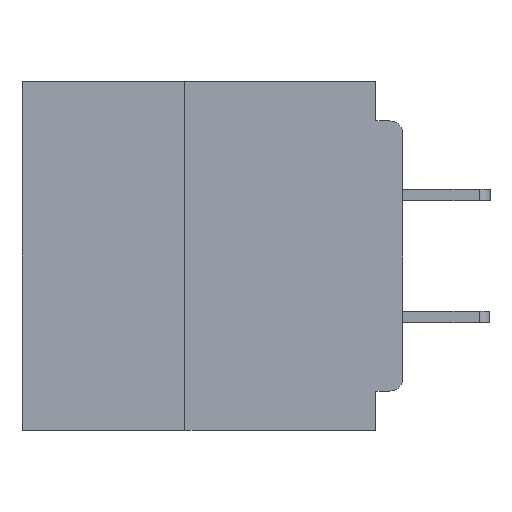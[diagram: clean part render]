
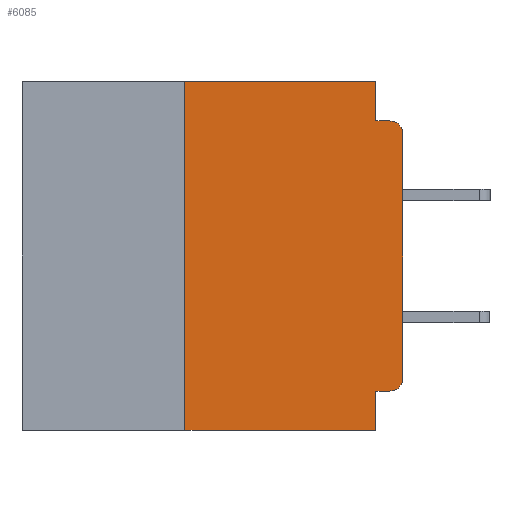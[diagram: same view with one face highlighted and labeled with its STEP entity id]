
A CAD part, left-side view. The second image highlights one B-rep face of the part: STEP entity #6085.
In plain terms, the highlighted planar face has unit normal (-1, 0, 0).
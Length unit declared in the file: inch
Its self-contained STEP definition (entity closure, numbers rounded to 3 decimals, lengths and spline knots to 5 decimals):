
#209 = LINE ( 'NONE', #24996, #17681 ) ;
#432 = CARTESIAN_POINT ( 'NONE',  ( 0., 0.015, -0.045 ) ) ;
#814 = VECTOR ( 'NONE', #6378, 39.37008 ) ;
#1508 = EDGE_CURVE ( 'NONE', #24689, #15561, #11261, .T. ) ;
#1944 = EDGE_CURVE ( 'NONE', #20223, #42986, #40519, .T. ) ;
#2173 = VECTOR ( 'NONE', #44074, 39.37008 ) ;
#2758 = CARTESIAN_POINT ( 'NONE',  ( 0., 0.437, -0.4 ) ) ;
#2955 = CARTESIAN_POINT ( 'NONE',  ( 0., 0.015, -0.355 ) ) ;
#4471 = VECTOR ( 'NONE', #29755, 39.37008 ) ;
#5845 = CARTESIAN_POINT ( 'NONE',  ( 0., 0.25, 0. ) ) ;
#6073 = CARTESIAN_POINT ( 'NONE',  ( 0., 0.015, -0.06 ) ) ;
#6085 = ADVANCED_FACE ( 'NONE', ( #31059 ), #6500, .F. ) ;
#6378 = DIRECTION ( 'NONE',  ( 0., 1., 0. ) ) ;
#6500 = PLANE ( 'NONE',  #25176 ) ;
#6593 = CARTESIAN_POINT ( 'NONE',  ( 0., 0., -0.355 ) ) ;
#7092 = LINE ( 'NONE', #2758, #25419 ) ;
#7213 = ORIENTED_EDGE ( 'NONE', *, *, #21589, .T. ) ;
#7662 = CARTESIAN_POINT ( 'NONE',  ( 0., 0., -0.06 ) ) ;
#9269 = CARTESIAN_POINT ( 'NONE',  ( 0., 0.437, 0. ) ) ;
#9565 = DIRECTION ( 'NONE',  ( 0., 0., -1. ) ) ;
#9744 = CIRCLE ( 'NONE', #31166, 0.015 ) ;
#9876 = VERTEX_POINT ( 'NONE', #36592 ) ;
#9993 = DIRECTION ( 'NONE',  ( 1., 0., 0. ) ) ;
#10496 = EDGE_CURVE ( 'NONE', #26875, #34018, #22851, .T. ) ;
#11261 = LINE ( 'NONE', #6593, #814 ) ;
#11410 = EDGE_CURVE ( 'NONE', #15561, #9876, #30737, .T. ) ;
#11480 = LINE ( 'NONE', #43930, #2173 ) ;
#12088 = VECTOR ( 'NONE', #33208, 39.37008 ) ;
#15561 = VERTEX_POINT ( 'NONE', #44194 ) ;
#16716 = DIRECTION ( 'NONE',  ( 0., 0., -1. ) ) ;
#17394 = VERTEX_POINT ( 'NONE', #41578 ) ;
#17456 = EDGE_CURVE ( 'NONE', #17394, #35552, #209, .T. ) ;
#17681 = VECTOR ( 'NONE', #28429, 39.37008 ) ;
#19764 = EDGE_CURVE ( 'NONE', #35552, #20223, #30267, .T. ) ;
#20223 = VERTEX_POINT ( 'NONE', #32751 ) ;
#20227 = CARTESIAN_POINT ( 'NONE',  ( 0., 0.437, 0. ) ) ;
#20500 = CARTESIAN_POINT ( 'NONE',  ( 0., 0.015, -0.34 ) ) ;
#20991 = EDGE_CURVE ( 'NONE', #17394, #9876, #7092, .T. ) ;
#21589 = EDGE_CURVE ( 'NONE', #34018, #39240, #9744, .T. ) ;
#21604 = CARTESIAN_POINT ( 'NONE',  ( 0., 0.031, 0. ) ) ;
#22851 = LINE ( 'NONE', #43211, #4471 ) ;
#23958 = DIRECTION ( 'NONE',  ( 0., 0., -1. ) ) ;
#24314 = AXIS2_PLACEMENT_3D ( 'NONE', #20500, #44247, #23958 ) ;
#24689 = VERTEX_POINT ( 'NONE', #2955 ) ;
#24996 = CARTESIAN_POINT ( 'NONE',  ( 0., 0.25, -0.4 ) ) ;
#25176 = AXIS2_PLACEMENT_3D ( 'NONE', #20227, #9993, #33913 ) ;
#25419 = VECTOR ( 'NONE', #36936, 39.37008 ) ;
#26376 = CIRCLE ( 'NONE', #24314, 0.015 ) ;
#26875 = VERTEX_POINT ( 'NONE', #36315 ) ;
#27724 = CARTESIAN_POINT ( 'NONE',  ( 0., 0.031, -0.045 ) ) ;
#27869 = ORIENTED_EDGE ( 'NONE', *, *, #20991, .T. ) ;
#27899 = ORIENTED_EDGE ( 'NONE', *, *, #1944, .F. ) ;
#28429 = DIRECTION ( 'NONE',  ( 0., 0., 1. ) ) ;
#29681 = VECTOR ( 'NONE', #16716, 39.37008 ) ;
#29755 = DIRECTION ( 'NONE',  ( 0., 0., 1. ) ) ;
#30113 = DIRECTION ( 'NONE',  ( -1., 0., 0. ) ) ;
#30267 = LINE ( 'NONE', #9269, #12088 ) ;
#30483 = VECTOR ( 'NONE', #41935, 39.37008 ) ;
#30646 = EDGE_CURVE ( 'NONE', #42986, #39240, #11480, .T. ) ;
#30737 = LINE ( 'NONE', #43900, #29681 ) ;
#31059 = FACE_OUTER_BOUND ( 'NONE', #42740, .T. ) ;
#31166 = AXIS2_PLACEMENT_3D ( 'NONE', #6073, #30113, #9565 ) ;
#32751 = CARTESIAN_POINT ( 'NONE',  ( 0., 0.031, 0. ) ) ;
#33208 = DIRECTION ( 'NONE',  ( 0., -1., 0. ) ) ;
#33913 = DIRECTION ( 'NONE',  ( 0., 0., -1. ) ) ;
#34018 = VERTEX_POINT ( 'NONE', #7662 ) ;
#35078 = ORIENTED_EDGE ( 'NONE', *, *, #17456, .F. ) ;
#35552 = VERTEX_POINT ( 'NONE', #5845 ) ;
#36315 = CARTESIAN_POINT ( 'NONE',  ( 0., 0., -0.34 ) ) ;
#36592 = CARTESIAN_POINT ( 'NONE',  ( 0., 0.031, -0.4 ) ) ;
#36936 = DIRECTION ( 'NONE',  ( 0., -1., 0. ) ) ;
#37521 = ORIENTED_EDGE ( 'NONE', *, *, #10496, .T. ) ;
#37665 = ORIENTED_EDGE ( 'NONE', *, *, #40474, .T. ) ;
#39240 = VERTEX_POINT ( 'NONE', #432 ) ;
#39669 = ORIENTED_EDGE ( 'NONE', *, *, #19764, .F. ) ;
#40474 = EDGE_CURVE ( 'NONE', #24689, #26875, #26376, .T. ) ;
#40519 = LINE ( 'NONE', #21604, #30483 ) ;
#40814 = ORIENTED_EDGE ( 'NONE', *, *, #11410, .F. ) ;
#41536 = ORIENTED_EDGE ( 'NONE', *, *, #30646, .F. ) ;
#41578 = CARTESIAN_POINT ( 'NONE',  ( 0., 0.25, -0.4 ) ) ;
#41935 = DIRECTION ( 'NONE',  ( 0., 0., -1. ) ) ;
#42740 = EDGE_LOOP ( 'NONE', ( #37521, #7213, #41536, #27899, #39669, #35078, #27869, #40814, #43557, #37665 ) ) ;
#42986 = VERTEX_POINT ( 'NONE', #27724 ) ;
#43211 = CARTESIAN_POINT ( 'NONE',  ( 0., 0., 0. ) ) ;
#43557 = ORIENTED_EDGE ( 'NONE', *, *, #1508, .F. ) ;
#43900 = CARTESIAN_POINT ( 'NONE',  ( 0., 0.031, -0.4 ) ) ;
#43930 = CARTESIAN_POINT ( 'NONE',  ( 0., 0., -0.045 ) ) ;
#44074 = DIRECTION ( 'NONE',  ( 0., -1., 0. ) ) ;
#44194 = CARTESIAN_POINT ( 'NONE',  ( 0., 0.031, -0.355 ) ) ;
#44247 = DIRECTION ( 'NONE',  ( -1., 0., 0. ) ) ;
